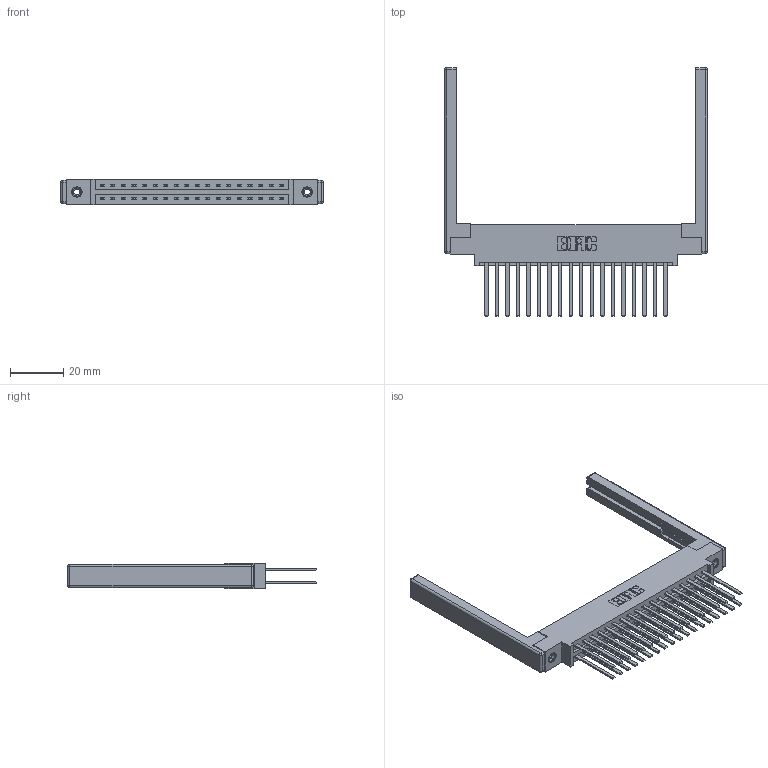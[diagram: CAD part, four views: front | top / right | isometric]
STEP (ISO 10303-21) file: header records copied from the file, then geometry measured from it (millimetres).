
FILE_DESCRIPTION (( 'STEP AP203' ), '1' );
FILE_NAME ('387-036-544-868.STEP', '2019-10-17T19:48:07', ( '' ), ( '' ), 'SwSTEP 2.0', 'SolidWorks 2016', '' );
FILE_SCHEMA (( 'CONFIG_CONTROL_DESIGN' ));
Length unit declared in the file: inch
Products named in the file (5): 337 Part_0.170 Offset - 0.156 Dia-TI; 307-220-068; 345-292-001_345-293-144; 387-036-544-868; 345-250-001_345-250-001-102
Assembly tree (41 placements, depth 2):
  387-036-544-868
    337 Part_0.170 Offset - 0.156 Dia-TI
    345-292-001_345-293-144  x36
    345-250-001_345-250-001-102  x2
    307-220-068  x2
Bounding box: 98.76 x 93.35 x 9.4 mm (x, y, z)
Volume: 14860.1 mm3; surface area: 17400 mm2
Topology: 41 solids, 41 shells, 2000 faces, 5861 edges, 3838 vertices
Faces by surface type: plane 1386, cylinder 590, cone 12, sphere 8, torus 4
Entity records: 19768 total; most frequent: CARTESIAN_POINT 3315, ORIENTED_EDGE 3240, DIRECTION 2930, EDGE_CURVE 1620, VECTOR 1446, LINE 1446, VERTEX_POINT 1070, AXIS2_PLACEMENT_3D 742
